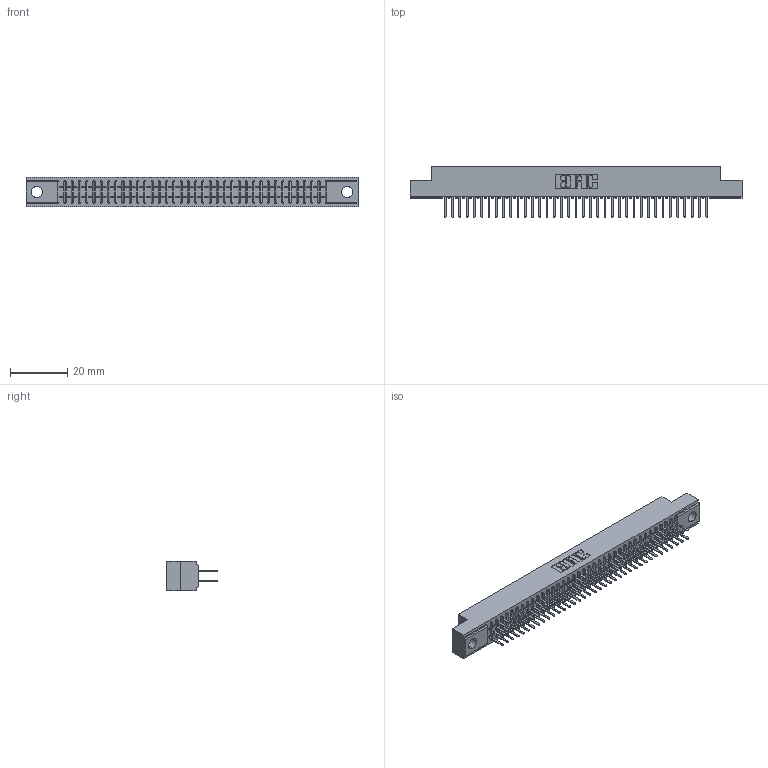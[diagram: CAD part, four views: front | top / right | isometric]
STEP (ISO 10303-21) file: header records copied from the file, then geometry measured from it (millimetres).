
FILE_DESCRIPTION (( 'STEP AP203' ), '1' );
FILE_NAME ('391-074-521-204.STEP', '2018-08-09T14:37:33', ( '' ), ( '' ), 'SwSTEP 2.0', 'SolidWorks 2016', '' );
FILE_SCHEMA (( 'CONFIG_CONTROL_DESIGN' ));
Length unit declared in the file: inch
Products named in the file (3): 341 Part_.156 (3.96) Dia Mounting Holes; 341-292-001_341-292-121; 391-074-521-204
Assembly tree (75 placements, depth 2):
  391-074-521-204
    341 Part_.156 (3.96) Dia Mounting Holes
    341-292-001_341-292-121  x74
Bounding box: 116.2 x 17.7 x 10.16 mm (x, y, z)
Volume: 8526.9 mm3; surface area: 15190.8 mm2
Topology: 75 solids, 75 shells, 5014 faces, 14523 edges, 9406 vertices
Faces by surface type: plane 3042, cylinder 1824, sphere 76, torus 72
Entity records: 45862 total; most frequent: CARTESIAN_POINT 7629, ORIENTED_EDGE 7578, DIRECTION 7399, EDGE_CURVE 3789, LINE 3063, VECTOR 3063, VERTEX_POINT 2398, AXIS2_PLACEMENT_3D 2168
